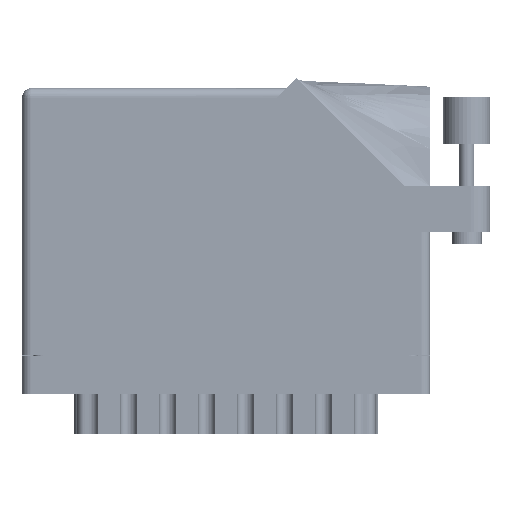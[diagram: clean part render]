
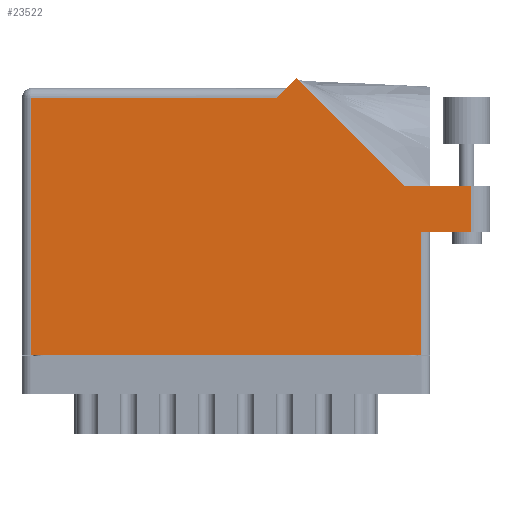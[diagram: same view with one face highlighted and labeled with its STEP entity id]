
A CAD part, front view. The second image highlights one B-rep face of the part: STEP entity #23522.
In plain terms, the highlighted face is planar.
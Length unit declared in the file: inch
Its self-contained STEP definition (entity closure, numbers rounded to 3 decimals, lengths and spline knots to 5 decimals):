
#272 = CARTESIAN_POINT ( 'NONE',  ( 2.993, 1.122, 0. ) ) ;
#623 = LINE ( 'NONE', #73464, #61643 ) ;
#690 = EDGE_CURVE ( 'NONE', #18753, #64054, #623, .T. ) ;
#1081 = EDGE_CURVE ( 'NONE', #75117, #18753, #33607, .T. ) ;
#3279 = VECTOR ( 'NONE', #44565, 39.37008 ) ;
#3442 = FACE_OUTER_BOUND ( 'NONE', #33210, .T. ) ;
#3516 = ORIENTED_EDGE ( 'NONE', *, *, #65046, .T. ) ;
#3900 = CARTESIAN_POINT ( 'NONE',  ( 0., 1.775, 0. ) ) ;
#6262 = DIRECTION ( 'NONE',  ( -1., 0., 0. ) ) ;
#7945 = VECTOR ( 'NONE', #48073, 39.37008 ) ;
#8593 = CARTESIAN_POINT ( 'NONE',  ( 2.993, 1.122, 0. ) ) ;
#8821 = LINE ( 'NONE', #45703, #53233 ) ;
#11703 = LINE ( 'NONE', #33466, #45022 ) ;
#13256 = CARTESIAN_POINT ( 'NONE',  ( 0.062, 0., 0. ) ) ;
#15865 = ORIENTED_EDGE ( 'NONE', *, *, #25480, .T. ) ;
#15921 = ORIENTED_EDGE ( 'NONE', *, *, #690, .T. ) ;
#16620 = VERTEX_POINT ( 'NONE', #63548 ) ;
#16971 = ORIENTED_EDGE ( 'NONE', *, *, #60284, .T. ) ;
#18189 = CARTESIAN_POINT ( 'NONE',  ( 0., 1.713, 0. ) ) ;
#18573 = ORIENTED_EDGE ( 'NONE', *, *, #59104, .T. ) ;
#18753 = VERTEX_POINT ( 'NONE', #57398 ) ;
#20667 = VECTOR ( 'NONE', #6262, 39.37008 ) ;
#23522 = ADVANCED_FACE ( 'NONE', ( #3442 ), #38399, .F. ) ;
#23790 = VERTEX_POINT ( 'NONE', #272 ) ;
#24368 = EDGE_CURVE ( 'NONE', #62387, #35246, #8821, .T. ) ;
#24661 = LINE ( 'NONE', #31866, #7945 ) ;
#25285 = ORIENTED_EDGE ( 'NONE', *, *, #24368, .T. ) ;
#25480 = EDGE_CURVE ( 'NONE', #55341, #16620, #69663, .T. ) ;
#27775 = DIRECTION ( 'NONE',  ( 1., 0., 0. ) ) ;
#30001 = VECTOR ( 'NONE', #74386, 39.37008 ) ;
#31866 = CARTESIAN_POINT ( 'NONE',  ( 3.118, 1.122, 0. ) ) ;
#32867 = EDGE_CURVE ( 'NONE', #23790, #55341, #24661, .T. ) ;
#33184 = DIRECTION ( 'NONE',  ( 0., 0., -1. ) ) ;
#33210 = EDGE_LOOP ( 'NONE', ( #25285, #3516, #50289, #15865, #60298, #33505, #15921, #16971, #18573 ) ) ;
#33466 = CARTESIAN_POINT ( 'NONE',  ( 0., 0., 0. ) ) ;
#33505 = ORIENTED_EDGE ( 'NONE', *, *, #1081, .T. ) ;
#33607 = LINE ( 'NONE', #18189, #20667 ) ;
#33670 = CARTESIAN_POINT ( 'NONE',  ( 2.55242, 1.122, 0. ) ) ;
#33693 = EDGE_CURVE ( 'NONE', #16620, #75117, #55121, .T. ) ;
#35246 = VERTEX_POINT ( 'NONE', #41984 ) ;
#37772 = LINE ( 'NONE', #39076, #62580 ) ;
#38091 = CARTESIAN_POINT ( 'NONE',  ( 2.656, 0.815, 0. ) ) ;
#38399 = PLANE ( 'NONE',  #58972 ) ;
#39076 = CARTESIAN_POINT ( 'NONE',  ( 2.656, 0.815, 0. ) ) ;
#41984 = CARTESIAN_POINT ( 'NONE',  ( 2.993, 0.815, 0. ) ) ;
#43325 = CARTESIAN_POINT ( 'NONE',  ( 2.656, 0., 0. ) ) ;
#44565 = DIRECTION ( 'NONE',  ( 0., 1., 0. ) ) ;
#45022 = VECTOR ( 'NONE', #27775, 39.37008 ) ;
#45703 = CARTESIAN_POINT ( 'NONE',  ( 2.718, 0.815, 0. ) ) ;
#48073 = DIRECTION ( 'NONE',  ( -1., 0., 0. ) ) ;
#49184 = VERTEX_POINT ( 'NONE', #43325 ) ;
#50289 = ORIENTED_EDGE ( 'NONE', *, *, #32867, .T. ) ;
#51426 = VECTOR ( 'NONE', #68544, 39.37008 ) ;
#53233 = VECTOR ( 'NONE', #63966, 39.37008 ) ;
#55121 = LINE ( 'NONE', #75472, #51426 ) ;
#55341 = VERTEX_POINT ( 'NONE', #57883 ) ;
#57398 = CARTESIAN_POINT ( 'NONE',  ( 0.062, 1.713, 0. ) ) ;
#57883 = CARTESIAN_POINT ( 'NONE',  ( 2.55242, 1.122, 0. ) ) ;
#58972 = AXIS2_PLACEMENT_3D ( 'NONE', #3900, #33184, #73657 ) ;
#59104 = EDGE_CURVE ( 'NONE', #49184, #62387, #37772, .T. ) ;
#60284 = EDGE_CURVE ( 'NONE', #64054, #49184, #11703, .T. ) ;
#60298 = ORIENTED_EDGE ( 'NONE', *, *, #33693, .T. ) ;
#61643 = VECTOR ( 'NONE', #62131, 39.37008 ) ;
#62131 = DIRECTION ( 'NONE',  ( 0., -1., 0. ) ) ;
#62387 = VERTEX_POINT ( 'NONE', #38091 ) ;
#62580 = VECTOR ( 'NONE', #74851, 39.37008 ) ;
#63318 = LINE ( 'NONE', #8593, #3279 ) ;
#63548 = CARTESIAN_POINT ( 'NONE',  ( 1.82871, 1.84571, 0. ) ) ;
#63966 = DIRECTION ( 'NONE',  ( 1., 0., 0. ) ) ;
#64054 = VERTEX_POINT ( 'NONE', #13256 ) ;
#65046 = EDGE_CURVE ( 'NONE', #35246, #23790, #63318, .T. ) ;
#68544 = DIRECTION ( 'NONE',  ( -0.707, -0.707, 0. ) ) ;
#69663 = LINE ( 'NONE', #33670, #30001 ) ;
#73464 = CARTESIAN_POINT ( 'NONE',  ( 0.062, 0., 0. ) ) ;
#73657 = DIRECTION ( 'NONE',  ( -1., 0., 0. ) ) ;
#74293 = CARTESIAN_POINT ( 'NONE',  ( 1.696, 1.713, 0. ) ) ;
#74386 = DIRECTION ( 'NONE',  ( -0.707, 0.707, 0. ) ) ;
#74851 = DIRECTION ( 'NONE',  ( 0., 1., 0. ) ) ;
#75117 = VERTEX_POINT ( 'NONE', #74293 ) ;
#75472 = CARTESIAN_POINT ( 'NONE',  ( 1.758, 1.775, 0. ) ) ;
